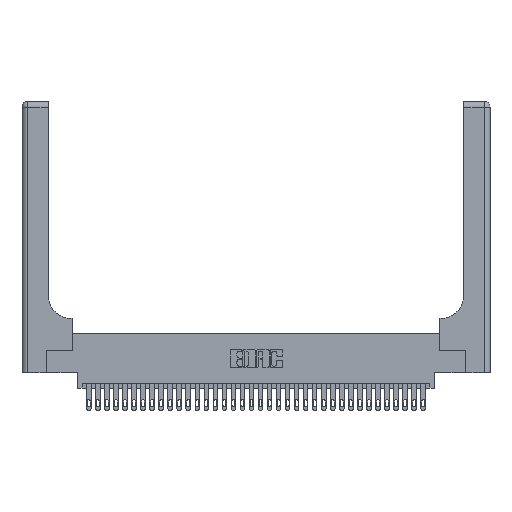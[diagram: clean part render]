
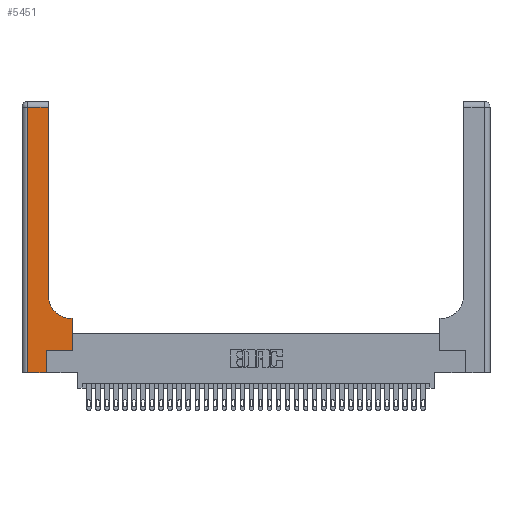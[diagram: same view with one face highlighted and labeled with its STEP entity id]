
A CAD part, top view. The second image highlights one B-rep face of the part: STEP entity #5451.
In plain terms, the highlighted planar face has unit normal (0, 0, 1).
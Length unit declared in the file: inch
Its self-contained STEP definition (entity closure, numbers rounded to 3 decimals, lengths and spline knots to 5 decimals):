
#138 = VECTOR ( 'NONE', #28888, 39.37008 ) ;
#274 = EDGE_CURVE ( 'NONE', #6649, #4099, #13822, .T. ) ;
#496 = CARTESIAN_POINT ( 'NONE',  ( 0.269, 0., 0.37 ) ) ;
#1438 = CARTESIAN_POINT ( 'NONE',  ( 0.5585, 0.6, 0.37 ) ) ;
#1576 = CARTESIAN_POINT ( 'NONE',  ( 0.269, 0.25, 0.37 ) ) ;
#2306 = VERTEX_POINT ( 'NONE', #25292 ) ;
#2618 = LINE ( 'NONE', #8075, #15574 ) ;
#2747 = EDGE_LOOP ( 'NONE', ( #27620, #3930, #11044, #14800, #14989, #8669, #17042, #3454, #29280 ) ) ;
#3454 = ORIENTED_EDGE ( 'NONE', *, *, #22031, .T. ) ;
#3930 = ORIENTED_EDGE ( 'NONE', *, *, #27342, .T. ) ;
#4099 = VERTEX_POINT ( 'NONE', #18519 ) ;
#4524 = DIRECTION ( 'NONE',  ( 0., 0., -1. ) ) ;
#4919 = VECTOR ( 'NONE', #7017, 39.37008 ) ;
#5451 = ADVANCED_FACE ( 'NONE', ( #10296 ), #9979, .F. ) ;
#6649 = VERTEX_POINT ( 'NONE', #19110 ) ;
#7017 = DIRECTION ( 'NONE',  ( 1., 0., 0. ) ) ;
#7604 = VERTEX_POINT ( 'NONE', #13490 ) ;
#8075 = CARTESIAN_POINT ( 'NONE',  ( 0.06, 3., 0.37 ) ) ;
#8669 = ORIENTED_EDGE ( 'NONE', *, *, #14669, .T. ) ;
#8862 = EDGE_CURVE ( 'NONE', #2306, #34570, #18497, .T. ) ;
#9248 = VECTOR ( 'NONE', #24525, 39.37008 ) ;
#9738 = DIRECTION ( 'NONE',  ( -1., 0., 0. ) ) ;
#9979 = PLANE ( 'NONE',  #29817 ) ;
#10036 = VERTEX_POINT ( 'NONE', #16244 ) ;
#10296 = FACE_OUTER_BOUND ( 'NONE', #2747, .T. ) ;
#11044 = ORIENTED_EDGE ( 'NONE', *, *, #24560, .T. ) ;
#13046 = EDGE_CURVE ( 'NONE', #4099, #7604, #31155, .T. ) ;
#13116 = VERTEX_POINT ( 'NONE', #15666 ) ;
#13490 = CARTESIAN_POINT ( 'NONE',  ( 0.2915, 2.94, 0.37 ) ) ;
#13822 = CIRCLE ( 'NONE', #19299, 0.25 ) ;
#14669 = EDGE_CURVE ( 'NONE', #10036, #2306, #35421, .T. ) ;
#14800 = ORIENTED_EDGE ( 'NONE', *, *, #20556, .T. ) ;
#14989 = ORIENTED_EDGE ( 'NONE', *, *, #19679, .T. ) ;
#15574 = VECTOR ( 'NONE', #21963, 39.37008 ) ;
#15666 = CARTESIAN_POINT ( 'NONE',  ( 0.269, 0., 0.37 ) ) ;
#16244 = CARTESIAN_POINT ( 'NONE',  ( 0.269, 0.25, 0.37 ) ) ;
#16722 = CARTESIAN_POINT ( 'NONE',  ( 0.5585, 0.25, 0.37 ) ) ;
#16740 = DIRECTION ( 'NONE',  ( -1., 0., 0. ) ) ;
#17042 = ORIENTED_EDGE ( 'NONE', *, *, #8862, .T. ) ;
#17991 = DIRECTION ( 'NONE',  ( 1., 0., 0. ) ) ;
#18497 = LINE ( 'NONE', #16722, #21935 ) ;
#18519 = CARTESIAN_POINT ( 'NONE',  ( 0.2915, 0.85, 0.37 ) ) ;
#19002 = CARTESIAN_POINT ( 'NONE',  ( 0.06, 0., 0.37 ) ) ;
#19110 = CARTESIAN_POINT ( 'NONE',  ( 0.5415, 0.6, 0.37 ) ) ;
#19299 = AXIS2_PLACEMENT_3D ( 'NONE', #32871, #24668, #22376 ) ;
#19486 = CARTESIAN_POINT ( 'NONE',  ( 0., 2.94, 0.37 ) ) ;
#19679 = EDGE_CURVE ( 'NONE', #13116, #10036, #26515, .T. ) ;
#19715 = DIRECTION ( 'NONE',  ( 0., 1., 0. ) ) ;
#20556 = EDGE_CURVE ( 'NONE', #28502, #13116, #20932, .T. ) ;
#20922 = VECTOR ( 'NONE', #19715, 39.37008 ) ;
#20932 = LINE ( 'NONE', #21348, #33823 ) ;
#21348 = CARTESIAN_POINT ( 'NONE',  ( 0., 0., 0.37 ) ) ;
#21935 = VECTOR ( 'NONE', #22117, 39.37008 ) ;
#21963 = DIRECTION ( 'NONE',  ( 0., -1., 0. ) ) ;
#22031 = EDGE_CURVE ( 'NONE', #34570, #6649, #25973, .T. ) ;
#22117 = DIRECTION ( 'NONE',  ( 0., 1., 0. ) ) ;
#22266 = VECTOR ( 'NONE', #16740, 39.37008 ) ;
#22376 = DIRECTION ( 'NONE',  ( 1., 0., 0. ) ) ;
#23344 = CARTESIAN_POINT ( 'NONE',  ( 0.2915, 3., 0.37 ) ) ;
#23560 = LINE ( 'NONE', #19486, #22266 ) ;
#24525 = DIRECTION ( 'NONE',  ( -1., 0., 0. ) ) ;
#24560 = EDGE_CURVE ( 'NONE', #24659, #28502, #2618, .T. ) ;
#24659 = VERTEX_POINT ( 'NONE', #27634 ) ;
#24668 = DIRECTION ( 'NONE',  ( 0., 0., -1. ) ) ;
#25292 = CARTESIAN_POINT ( 'NONE',  ( 0.5585, 0.25, 0.37 ) ) ;
#25973 = LINE ( 'NONE', #33189, #9248 ) ;
#26515 = LINE ( 'NONE', #496, #20922 ) ;
#27342 = EDGE_CURVE ( 'NONE', #7604, #24659, #23560, .T. ) ;
#27620 = ORIENTED_EDGE ( 'NONE', *, *, #13046, .T. ) ;
#27634 = CARTESIAN_POINT ( 'NONE',  ( 0.06, 2.94, 0.37 ) ) ;
#28502 = VERTEX_POINT ( 'NONE', #19002 ) ;
#28828 = CARTESIAN_POINT ( 'NONE',  ( 0., 3., 0.37 ) ) ;
#28888 = DIRECTION ( 'NONE',  ( 0., 1., 0. ) ) ;
#29280 = ORIENTED_EDGE ( 'NONE', *, *, #274, .T. ) ;
#29817 = AXIS2_PLACEMENT_3D ( 'NONE', #28828, #4524, #9738 ) ;
#31155 = LINE ( 'NONE', #23344, #138 ) ;
#32871 = CARTESIAN_POINT ( 'NONE',  ( 0.5415, 0.85, 0.37 ) ) ;
#33189 = CARTESIAN_POINT ( 'NONE',  ( 0.2915, 0.6, 0.37 ) ) ;
#33823 = VECTOR ( 'NONE', #17991, 39.37008 ) ;
#34570 = VERTEX_POINT ( 'NONE', #1438 ) ;
#35421 = LINE ( 'NONE', #1576, #4919 ) ;
